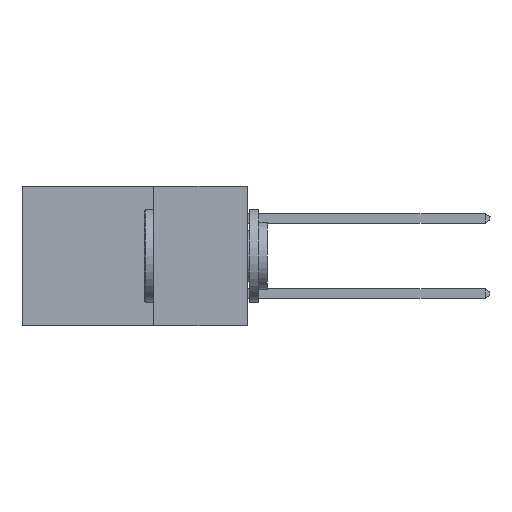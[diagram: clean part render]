
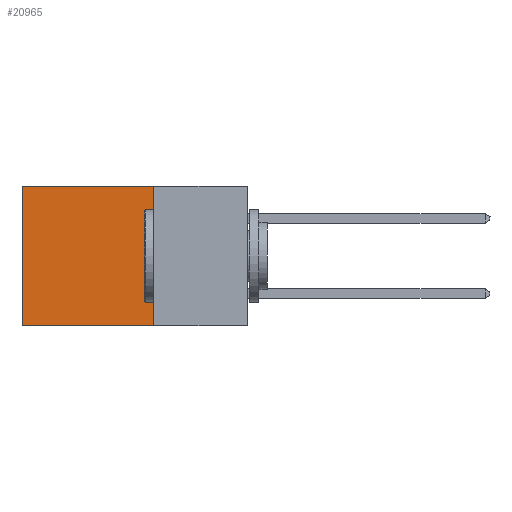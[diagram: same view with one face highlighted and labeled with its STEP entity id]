
A CAD part, left-side view. The second image highlights one B-rep face of the part: STEP entity #20965.
In plain terms, the highlighted planar face has unit normal (-1, 0, 0).
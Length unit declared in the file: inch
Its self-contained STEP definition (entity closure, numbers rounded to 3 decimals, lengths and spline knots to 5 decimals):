
#129 = EDGE_LOOP ( 'NONE', ( #9821, #17069, #16906, #19215 ) ) ;
#596 = EDGE_CURVE ( 'NONE', #2702, #20129, #9037, .T. ) ;
#2702 = VERTEX_POINT ( 'NONE', #10670 ) ;
#4181 = VECTOR ( 'NONE', #18388, 39.37008 ) ;
#4274 = AXIS2_PLACEMENT_3D ( 'NONE', #11226, #13096, #10903 ) ;
#4350 = VECTOR ( 'NONE', #21875, 39.37008 ) ;
#5070 = CARTESIAN_POINT ( 'NONE',  ( 0.298, 0.6, -0.37 ) ) ;
#9037 = LINE ( 'NONE', #20204, #4350 ) ;
#9267 = LINE ( 'NONE', #23220, #16569 ) ;
#9345 = PLANE ( 'NONE',  #4274 ) ;
#9821 = ORIENTED_EDGE ( 'NONE', *, *, #19609, .T. ) ;
#10670 = CARTESIAN_POINT ( 'NONE',  ( 0.298, 0.25, 0. ) ) ;
#10903 = DIRECTION ( 'NONE',  ( 0., 0., -1. ) ) ;
#11226 = CARTESIAN_POINT ( 'NONE',  ( 0.298, 0.25, 0. ) ) ;
#12526 = CARTESIAN_POINT ( 'NONE',  ( 0.298, 0.25, -0.37 ) ) ;
#12740 = CARTESIAN_POINT ( 'NONE',  ( 0.298, 0.6, 0. ) ) ;
#13096 = DIRECTION ( 'NONE',  ( 1., 0., 0. ) ) ;
#13810 = EDGE_CURVE ( 'NONE', #2702, #17891, #16136, .T. ) ;
#14480 = EDGE_CURVE ( 'NONE', #17891, #20059, #17688, .T. ) ;
#14489 = VECTOR ( 'NONE', #21796, 39.37008 ) ;
#15639 = DIRECTION ( 'NONE',  ( 0., 0., -1. ) ) ;
#15876 = FACE_OUTER_BOUND ( 'NONE', #129, .T. ) ;
#16136 = LINE ( 'NONE', #20051, #4181 ) ;
#16569 = VECTOR ( 'NONE', #15639, 39.37008 ) ;
#16906 = ORIENTED_EDGE ( 'NONE', *, *, #13810, .F. ) ;
#17069 = ORIENTED_EDGE ( 'NONE', *, *, #14480, .F. ) ;
#17688 = LINE ( 'NONE', #12526, #14489 ) ;
#17891 = VERTEX_POINT ( 'NONE', #23661 ) ;
#18388 = DIRECTION ( 'NONE',  ( 0., 0., -1. ) ) ;
#19215 = ORIENTED_EDGE ( 'NONE', *, *, #596, .T. ) ;
#19609 = EDGE_CURVE ( 'NONE', #20129, #20059, #9267, .T. ) ;
#20051 = CARTESIAN_POINT ( 'NONE',  ( 0.298, 0.25, 0. ) ) ;
#20059 = VERTEX_POINT ( 'NONE', #5070 ) ;
#20129 = VERTEX_POINT ( 'NONE', #12740 ) ;
#20204 = CARTESIAN_POINT ( 'NONE',  ( 0.298, 0.25, 0. ) ) ;
#20965 = ADVANCED_FACE ( 'NONE', ( #15876 ), #9345, .F. ) ;
#21796 = DIRECTION ( 'NONE',  ( 0., 1., 0. ) ) ;
#21875 = DIRECTION ( 'NONE',  ( 0., 1., 0. ) ) ;
#23220 = CARTESIAN_POINT ( 'NONE',  ( 0.298, 0.6, 0. ) ) ;
#23661 = CARTESIAN_POINT ( 'NONE',  ( 0.298, 0.25, -0.37 ) ) ;
